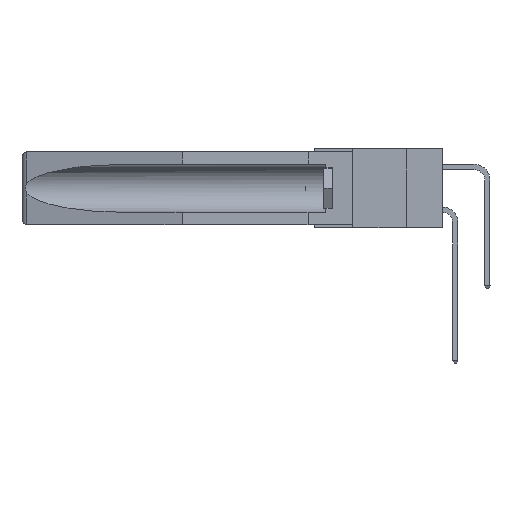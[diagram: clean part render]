
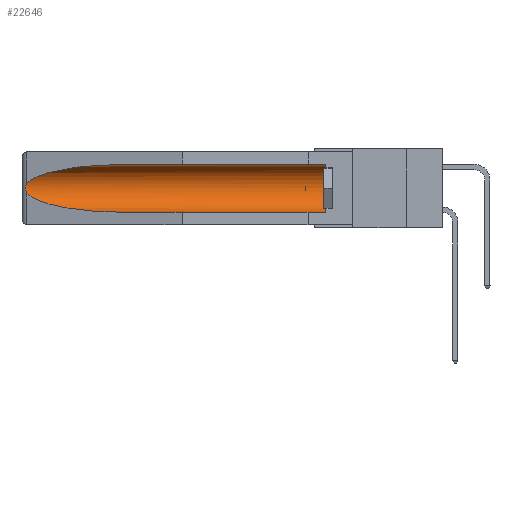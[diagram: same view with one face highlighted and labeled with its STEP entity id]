
A CAD part, left-side view. The second image highlights one B-rep face of the part: STEP entity #22646.
In plain terms, the highlighted cylindrical face has radius 2.857 mm (diameter 5.715 mm), a partial arc.
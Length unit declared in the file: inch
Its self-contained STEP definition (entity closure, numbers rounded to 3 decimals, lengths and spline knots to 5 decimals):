
#901 = CARTESIAN_POINT ( 'NONE',  ( 0.155, 1.07973, -0.059 ) ) ;
#1194 = CYLINDRICAL_SURFACE ( 'NONE', #31128, 0.1125 ) ;
#1556 = DIRECTION ( 'NONE',  ( 0., 1., 0. ) ) ;
#1626 = CARTESIAN_POINT ( 'NONE',  ( 0.155, 1.07973, -0.059 ) ) ;
#2652 = CARTESIAN_POINT ( 'NONE',  ( 0.2675, 1.53308, -0.17534 ) ) ;
#2860 = CARTESIAN_POINT ( 'NONE',  ( 0.155, 0.126, -0.059 ) ) ;
#3264 = DIRECTION ( 'NONE',  ( 0., 1., 0. ) ) ;
#4652 = EDGE_CURVE ( 'NONE', #23121, #11210, #10275, .T. ) ;
#5189 = CARTESIAN_POINT ( 'NONE',  ( 0.26654, 1.53092, -0.15636 ) ) ;
#5475 = ORIENTED_EDGE ( 'NONE', *, *, #25626, .T. ) ;
#7013 = LINE ( 'NONE', #23128, #17474 ) ;
#7300 = CARTESIAN_POINT ( 'NONE',  ( 0.155, 0.126, -0.1715 ) ) ;
#9563 = CARTESIAN_POINT ( 'NONE',  ( 0.26537, 1.52718, -0.19328 ) ) ;
#9925 = CARTESIAN_POINT ( 'NONE',  ( 0.21114, 1.30732, -0.059 ) ) ;
#9955 = LINE ( 'NONE', #17456, #18543 ) ;
#10275 = B_SPLINE_CURVE_WITH_KNOTS ( 'NONE', 3,
 ( #28522, #34657, #5189, #28394, #11186, #2652, #11064, #31454, #23056, #16878 ),
 .UNSPECIFIED., .F., .F.,
 ( 4, 2, 2, 2, 4 ),
 ( 0., 0.00029, 0.00058, 0.00087, 0.00117 ),
 .UNSPECIFIED. ) ;
#11064 = CARTESIAN_POINT ( 'NONE',  ( 0.2673, 1.53269, -0.17917 ) ) ;
#11155 = VERTEX_POINT ( 'NONE', #2860 ) ;
#11186 = CARTESIAN_POINT ( 'NONE',  ( 0.2675, 1.53308, -0.16763 ) ) ;
#11210 = VERTEX_POINT ( 'NONE', #9563 ) ;
#13224 = CIRCLE ( 'NONE', #33529, 0.1125 ) ;
#13554 = ORIENTED_EDGE ( 'NONE', *, *, #33506, .T. ) ;
#14040 = ORIENTED_EDGE ( 'NONE', *, *, #24365, .F. ) ;
#14535 = EDGE_CURVE ( 'NONE', #11155, #20878, #9955, .T. ) ;
#15082 = CARTESIAN_POINT ( 'NONE',  ( 0.155, 1.07973, -0.284 ) ) ;
#15323 = CARTESIAN_POINT ( 'NONE',  ( 0.155, 1.07973, -0.284 ) ) ;
#16059 = DIRECTION ( 'NONE',  ( 0., -1., 0. ) ) ;
#16369 = ORIENTED_EDGE ( 'NONE', *, *, #4652, .T. ) ;
#16660 = FACE_OUTER_BOUND ( 'NONE', #19760, .T. ) ;
#16878 = CARTESIAN_POINT ( 'NONE',  ( 0.26537, 1.52718, -0.19328 ) ) ;
#17392 = ORIENTED_EDGE ( 'NONE', *, *, #19524, .T. ) ;
#17456 = CARTESIAN_POINT ( 'NONE',  ( 0.155, -0.30754, -0.059 ) ) ;
#17474 = VECTOR ( 'NONE', #35088, 39.37008 ) ;
#18543 = VECTOR ( 'NONE', #3264, 39.37008 ) ;
#18633 = VERTEX_POINT ( 'NONE', #28869 ) ;
#18943 = DIRECTION ( 'NONE',  ( 0., 0., 1. ) ) ;
#19092 = DIRECTION ( 'NONE',  ( 0., 0., 1. ) ) ;
#19524 = EDGE_CURVE ( 'NONE', #18633, #11155, #13224, .T. ) ;
#19760 = EDGE_LOOP ( 'NONE', ( #5475, #16369, #13554, #14040, #17392, #26761 ) ) ;
#20157 = CARTESIAN_POINT ( 'NONE',  ( 0.25451, 1.48313, -0.24835 ) ) ;
#20878 = VERTEX_POINT ( 'NONE', #1626 ) ;
#22563 = CARTESIAN_POINT ( 'NONE',  ( 0.25451, 1.48313, -0.09465 ) ) ;
#22646 = ADVANCED_FACE ( 'NONE', ( #16660 ), #1194, .F. ) ;
#23056 = CARTESIAN_POINT ( 'NONE',  ( 0.26597, 1.5296, -0.19026 ) ) ;
#23121 = VERTEX_POINT ( 'NONE', #29137 ) ;
#23128 = CARTESIAN_POINT ( 'NONE',  ( 0.155, -0.30754, -0.284 ) ) ;
#24365 = EDGE_CURVE ( 'NONE', #18633, #33579, #7013, .T. ) ;
#25170 = CARTESIAN_POINT ( 'NONE',  ( 0.155, -0.30754, -0.1715 ) ) ;
#25600 =( BOUNDED_CURVE ( )  B_SPLINE_CURVE ( 3, ( #34872, #20157, #29501, #15323 ),
 .UNSPECIFIED., .F., .F. ) 
 B_SPLINE_CURVE_WITH_KNOTS ( ( 4, 4 ),
 ( 0.1948, 1.5708 ),
 .UNSPECIFIED. ) 
 CURVE ( )  GEOMETRIC_REPRESENTATION_ITEM ( )  RATIONAL_B_SPLINE_CURVE ( ( 1., 0.848, 0.848, 1. ) ) 
 REPRESENTATION_ITEM ( '' )  );
#25626 = EDGE_CURVE ( 'NONE', #20878, #23121, #30668, .T. ) ;
#26761 = ORIENTED_EDGE ( 'NONE', *, *, #14535, .T. ) ;
#28394 = CARTESIAN_POINT ( 'NONE',  ( 0.2673, 1.5327, -0.16383 ) ) ;
#28522 = CARTESIAN_POINT ( 'NONE',  ( 0.26537, 1.52718, -0.14972 ) ) ;
#28869 = CARTESIAN_POINT ( 'NONE',  ( 0.155, 0.126, -0.284 ) ) ;
#29137 = CARTESIAN_POINT ( 'NONE',  ( 0.26537, 1.52718, -0.14972 ) ) ;
#29501 = CARTESIAN_POINT ( 'NONE',  ( 0.21114, 1.30732, -0.284 ) ) ;
#30668 =( BOUNDED_CURVE ( )  B_SPLINE_CURVE ( 3, ( #901, #9925, #22563, #34778 ),
 .UNSPECIFIED., .F., .F. ) 
 B_SPLINE_CURVE_WITH_KNOTS ( ( 4, 4 ),
 ( 4.71239, 6.08839 ),
 .UNSPECIFIED. ) 
 CURVE ( )  GEOMETRIC_REPRESENTATION_ITEM ( )  RATIONAL_B_SPLINE_CURVE ( ( 1., 0.848, 0.848, 1. ) ) 
 REPRESENTATION_ITEM ( '' )  );
#31128 = AXIS2_PLACEMENT_3D ( 'NONE', #25170, #1556, #19092 ) ;
#31454 = CARTESIAN_POINT ( 'NONE',  ( 0.26655, 1.53094, -0.18657 ) ) ;
#33506 = EDGE_CURVE ( 'NONE', #11210, #33579, #25600, .T. ) ;
#33529 = AXIS2_PLACEMENT_3D ( 'NONE', #7300, #16059, #18943 ) ;
#33579 = VERTEX_POINT ( 'NONE', #15082 ) ;
#34657 = CARTESIAN_POINT ( 'NONE',  ( 0.26597, 1.52961, -0.15275 ) ) ;
#34778 = CARTESIAN_POINT ( 'NONE',  ( 0.26537, 1.52718, -0.14972 ) ) ;
#34872 = CARTESIAN_POINT ( 'NONE',  ( 0.26537, 1.52718, -0.19328 ) ) ;
#35088 = DIRECTION ( 'NONE',  ( 0., 1., 0. ) ) ;
